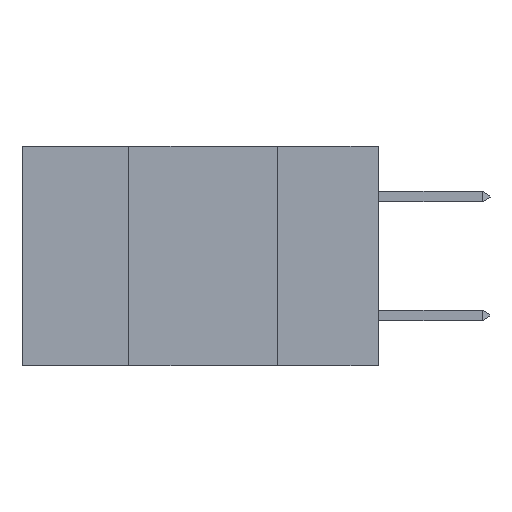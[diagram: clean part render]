
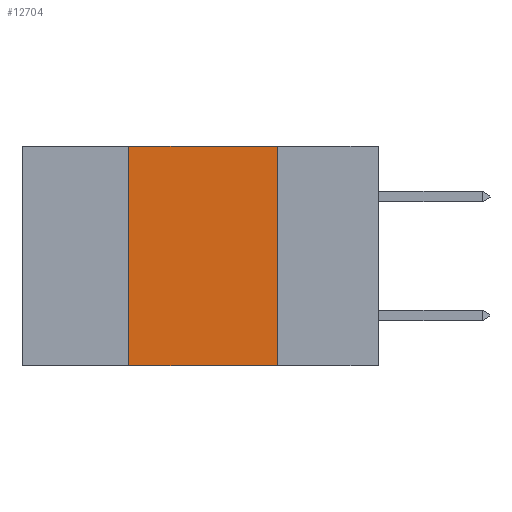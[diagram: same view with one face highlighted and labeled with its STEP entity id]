
A CAD part, left-side view. The second image highlights one B-rep face of the part: STEP entity #12704.
In plain terms, the highlighted planar face has unit normal (-1, 0, 0).
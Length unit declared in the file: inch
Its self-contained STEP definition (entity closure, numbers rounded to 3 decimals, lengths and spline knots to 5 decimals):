
#205 = DIRECTION ( 'NONE',  ( 0., -1., 0. ) ) ;
#1721 = ORIENTED_EDGE ( 'NONE', *, *, #16333, .F. ) ;
#2334 = DIRECTION ( 'NONE',  ( 0., 0., -1. ) ) ;
#2368 = VECTOR ( 'NONE', #12802, 39.37008 ) ;
#3883 = CARTESIAN_POINT ( 'NONE',  ( 0., 0.17, -0.37 ) ) ;
#4042 = CARTESIAN_POINT ( 'NONE',  ( 0., 0.17, 0. ) ) ;
#5289 = EDGE_CURVE ( 'NONE', #13143, #15082, #21891, .T. ) ;
#7144 = FACE_OUTER_BOUND ( 'NONE', #23028, .T. ) ;
#7226 = CARTESIAN_POINT ( 'NONE',  ( 0., 0.6, 0. ) ) ;
#8129 = DIRECTION ( 'NONE',  ( 0., 0., 1. ) ) ;
#8325 = ORIENTED_EDGE ( 'NONE', *, *, #9475, .T. ) ;
#8392 = VECTOR ( 'NONE', #8129, 39.37008 ) ;
#8913 = VECTOR ( 'NONE', #2334, 39.37008 ) ;
#9475 = EDGE_CURVE ( 'NONE', #20054, #15082, #13499, .T. ) ;
#11617 = LINE ( 'NONE', #19428, #8392 ) ;
#12704 = ADVANCED_FACE ( 'NONE', ( #7144 ), #20369, .F. ) ;
#12748 = ORIENTED_EDGE ( 'NONE', *, *, #18314, .F. ) ;
#12802 = DIRECTION ( 'NONE',  ( 0., -1., 0. ) ) ;
#13016 = LINE ( 'NONE', #14859, #2368 ) ;
#13143 = VERTEX_POINT ( 'NONE', #23035 ) ;
#13499 = LINE ( 'NONE', #16854, #14704 ) ;
#14477 = VERTEX_POINT ( 'NONE', #22751 ) ;
#14704 = VECTOR ( 'NONE', #205, 39.37008 ) ;
#14859 = CARTESIAN_POINT ( 'NONE',  ( 0., 0.6, 0. ) ) ;
#15082 = VERTEX_POINT ( 'NONE', #3883 ) ;
#16333 = EDGE_CURVE ( 'NONE', #20054, #14477, #11617, .T. ) ;
#16557 = DIRECTION ( 'NONE',  ( 1., 0., 0. ) ) ;
#16854 = CARTESIAN_POINT ( 'NONE',  ( 0., 0.6, -0.37 ) ) ;
#18314 = EDGE_CURVE ( 'NONE', #14477, #13143, #13016, .T. ) ;
#18830 = ORIENTED_EDGE ( 'NONE', *, *, #5289, .F. ) ;
#19428 = CARTESIAN_POINT ( 'NONE',  ( 0., 0.42, 0. ) ) ;
#20054 = VERTEX_POINT ( 'NONE', #20914 ) ;
#20369 = PLANE ( 'NONE',  #22974 ) ;
#20914 = CARTESIAN_POINT ( 'NONE',  ( 0., 0.42, -0.37 ) ) ;
#21891 = LINE ( 'NONE', #4042, #8913 ) ;
#22331 = DIRECTION ( 'NONE',  ( 0., 0., -1. ) ) ;
#22751 = CARTESIAN_POINT ( 'NONE',  ( 0., 0.42, 0. ) ) ;
#22974 = AXIS2_PLACEMENT_3D ( 'NONE', #7226, #16557, #22331 ) ;
#23028 = EDGE_LOOP ( 'NONE', ( #18830, #12748, #1721, #8325 ) ) ;
#23035 = CARTESIAN_POINT ( 'NONE',  ( 0., 0.17, 0. ) ) ;
